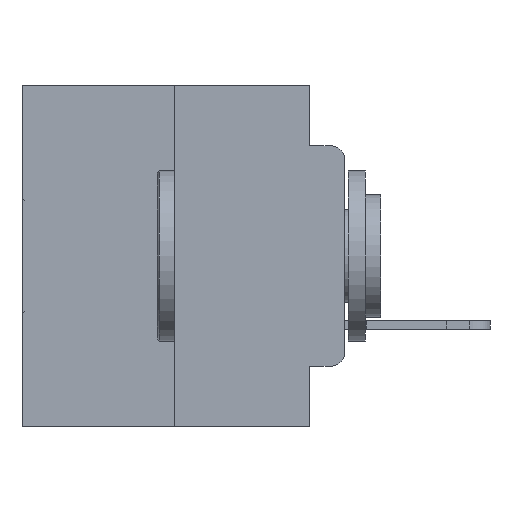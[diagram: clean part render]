
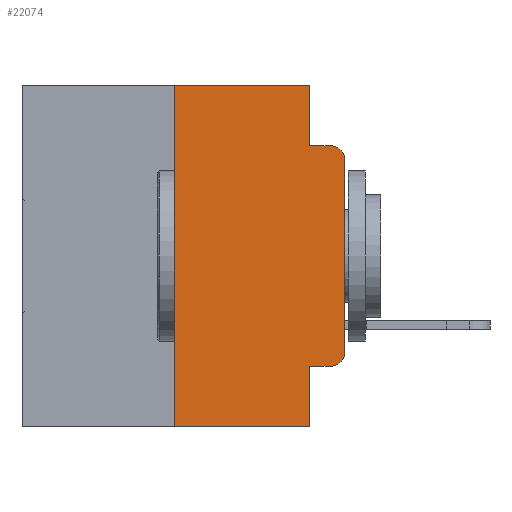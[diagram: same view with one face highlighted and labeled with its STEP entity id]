
A CAD part, left-side view. The second image highlights one B-rep face of the part: STEP entity #22074.
In plain terms, the highlighted planar face has unit normal (-1, 0, 0).
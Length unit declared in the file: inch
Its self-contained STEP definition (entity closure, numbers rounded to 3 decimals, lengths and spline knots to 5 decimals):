
#149 = VECTOR ( 'NONE', #12659, 39.37008 ) ;
#151 = VERTEX_POINT ( 'NONE', #11593 ) ;
#1165 = ORIENTED_EDGE ( 'NONE', *, *, #11433, .F. ) ;
#1255 = LINE ( 'NONE', #3064, #149 ) ;
#1271 = VERTEX_POINT ( 'NONE', #24097 ) ;
#1415 = DIRECTION ( 'NONE',  ( 0., 0., 1. ) ) ;
#1542 = DIRECTION ( 'NONE',  ( -1., 0., 0. ) ) ;
#1613 = CARTESIAN_POINT ( 'NONE',  ( 0., 0.051, 0. ) ) ;
#2626 = LINE ( 'NONE', #10739, #24595 ) ;
#3064 = CARTESIAN_POINT ( 'NONE',  ( 0., 0.051, -0.4115 ) ) ;
#3560 = LINE ( 'NONE', #21063, #25129 ) ;
#3998 = CARTESIAN_POINT ( 'NONE',  ( 0., 0.051, -0.5 ) ) ;
#4261 = VECTOR ( 'NONE', #7693, 39.37008 ) ;
#4513 = EDGE_CURVE ( 'NONE', #15420, #26045, #6459, .T. ) ;
#4899 = DIRECTION ( 'NONE',  ( 0., -1., 0. ) ) ;
#4928 = ORIENTED_EDGE ( 'NONE', *, *, #29384, .T. ) ;
#4986 = VECTOR ( 'NONE', #22672, 39.37008 ) ;
#5398 = CARTESIAN_POINT ( 'NONE',  ( 0., 0.25, 0. ) ) ;
#5448 = DIRECTION ( 'NONE',  ( 0., 0., -1. ) ) ;
#5647 = CARTESIAN_POINT ( 'NONE',  ( 0., 0.473, -0.5 ) ) ;
#5677 = LINE ( 'NONE', #5398, #4261 ) ;
#6052 = ORIENTED_EDGE ( 'NONE', *, *, #20696, .T. ) ;
#6459 = LINE ( 'NONE', #1613, #4986 ) ;
#6617 = CARTESIAN_POINT ( 'NONE',  ( 0., 0.473, 0. ) ) ;
#7275 = ORIENTED_EDGE ( 'NONE', *, *, #14151, .F. ) ;
#7693 = DIRECTION ( 'NONE',  ( 0., 0., 1. ) ) ;
#8144 = DIRECTION ( 'NONE',  ( 0., 0., -1. ) ) ;
#8159 = EDGE_CURVE ( 'NONE', #151, #26045, #21317, .T. ) ;
#8299 = EDGE_CURVE ( 'NONE', #23871, #17152, #2626, .T. ) ;
#8351 = CARTESIAN_POINT ( 'NONE',  ( 0., 0.02, -0.1085 ) ) ;
#9388 = CARTESIAN_POINT ( 'NONE',  ( 0., 0.473, 0. ) ) ;
#10129 = ORIENTED_EDGE ( 'NONE', *, *, #28683, .F. ) ;
#10229 = CARTESIAN_POINT ( 'NONE',  ( 0., 0.051, -0.4115 ) ) ;
#10248 = LINE ( 'NONE', #16850, #25395 ) ;
#10739 = CARTESIAN_POINT ( 'NONE',  ( 0., 0., 0. ) ) ;
#11229 = ORIENTED_EDGE ( 'NONE', *, *, #8299, .T. ) ;
#11433 = EDGE_CURVE ( 'NONE', #1271, #24642, #3560, .T. ) ;
#11593 = CARTESIAN_POINT ( 'NONE',  ( 0., 0.25, -0.5 ) ) ;
#12515 = DIRECTION ( 'NONE',  ( 0., -1., 0. ) ) ;
#12659 = DIRECTION ( 'NONE',  ( 0., -1., 0. ) ) ;
#13352 = AXIS2_PLACEMENT_3D ( 'NONE', #25929, #21676, #28217 ) ;
#13568 = DIRECTION ( 'NONE',  ( 1., 0., 0. ) ) ;
#13662 = DIRECTION ( 'NONE',  ( 0., 0., -1. ) ) ;
#13892 = CARTESIAN_POINT ( 'NONE',  ( 0., 0., -0.3915 ) ) ;
#14093 = LINE ( 'NONE', #9388, #25658 ) ;
#14151 = EDGE_CURVE ( 'NONE', #15032, #27181, #14093, .T. ) ;
#14369 = ORIENTED_EDGE ( 'NONE', *, *, #19771, .T. ) ;
#14909 = VERTEX_POINT ( 'NONE', #28778 ) ;
#15032 = VERTEX_POINT ( 'NONE', #26824 ) ;
#15093 = FACE_OUTER_BOUND ( 'NONE', #21423, .T. ) ;
#15420 = VERTEX_POINT ( 'NONE', #10229 ) ;
#16850 = CARTESIAN_POINT ( 'NONE',  ( 0., 0.051, 0. ) ) ;
#17152 = VERTEX_POINT ( 'NONE', #24539 ) ;
#18054 = PLANE ( 'NONE',  #26474 ) ;
#18361 = ORIENTED_EDGE ( 'NONE', *, *, #4513, .F. ) ;
#18419 = AXIS2_PLACEMENT_3D ( 'NONE', #8351, #1542, #8144 ) ;
#19771 = EDGE_CURVE ( 'NONE', #14909, #23871, #27203, .T. ) ;
#20696 = EDGE_CURVE ( 'NONE', #17152, #24642, #27810, .T. ) ;
#21063 = CARTESIAN_POINT ( 'NONE',  ( 0., 0.051, -0.0885 ) ) ;
#21317 = LINE ( 'NONE', #5647, #23488 ) ;
#21423 = EDGE_LOOP ( 'NONE', ( #11229, #6052, #1165, #10129, #7275, #26697, #21926, #18361, #4928, #14369 ) ) ;
#21676 = DIRECTION ( 'NONE',  ( -1., 0., 0. ) ) ;
#21926 = ORIENTED_EDGE ( 'NONE', *, *, #8159, .T. ) ;
#22074 = ADVANCED_FACE ( 'NONE', ( #15093 ), #18054, .F. ) ;
#22672 = DIRECTION ( 'NONE',  ( 0., 0., -1. ) ) ;
#23488 = VECTOR ( 'NONE', #12515, 39.37008 ) ;
#23871 = VERTEX_POINT ( 'NONE', #13892 ) ;
#24097 = CARTESIAN_POINT ( 'NONE',  ( 0., 0.051, -0.0885 ) ) ;
#24122 = CARTESIAN_POINT ( 'NONE',  ( 0., 0.051, 0. ) ) ;
#24168 = EDGE_CURVE ( 'NONE', #151, #15032, #5677, .T. ) ;
#24539 = CARTESIAN_POINT ( 'NONE',  ( 0., 0., -0.1085 ) ) ;
#24595 = VECTOR ( 'NONE', #1415, 39.37008 ) ;
#24642 = VERTEX_POINT ( 'NONE', #28134 ) ;
#25129 = VECTOR ( 'NONE', #25810, 39.37008 ) ;
#25395 = VECTOR ( 'NONE', #5448, 39.37008 ) ;
#25658 = VECTOR ( 'NONE', #4899, 39.37008 ) ;
#25810 = DIRECTION ( 'NONE',  ( 0., -1., 0. ) ) ;
#25929 = CARTESIAN_POINT ( 'NONE',  ( 0., 0.02, -0.3915 ) ) ;
#26045 = VERTEX_POINT ( 'NONE', #3998 ) ;
#26474 = AXIS2_PLACEMENT_3D ( 'NONE', #6617, #13568, #13662 ) ;
#26697 = ORIENTED_EDGE ( 'NONE', *, *, #24168, .F. ) ;
#26824 = CARTESIAN_POINT ( 'NONE',  ( 0., 0.25, 0. ) ) ;
#27181 = VERTEX_POINT ( 'NONE', #24122 ) ;
#27203 = CIRCLE ( 'NONE', #13352, 0.02 ) ;
#27810 = CIRCLE ( 'NONE', #18419, 0.02 ) ;
#28134 = CARTESIAN_POINT ( 'NONE',  ( 0., 0.02, -0.0885 ) ) ;
#28217 = DIRECTION ( 'NONE',  ( 0., 0., -1. ) ) ;
#28683 = EDGE_CURVE ( 'NONE', #27181, #1271, #10248, .T. ) ;
#28778 = CARTESIAN_POINT ( 'NONE',  ( 0., 0.02, -0.4115 ) ) ;
#29384 = EDGE_CURVE ( 'NONE', #15420, #14909, #1255, .T. ) ;
